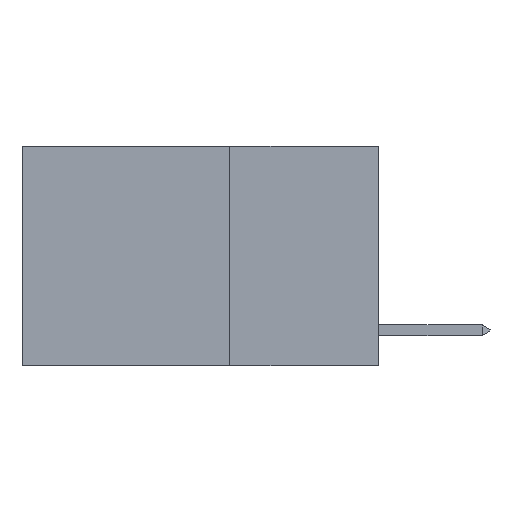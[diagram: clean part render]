
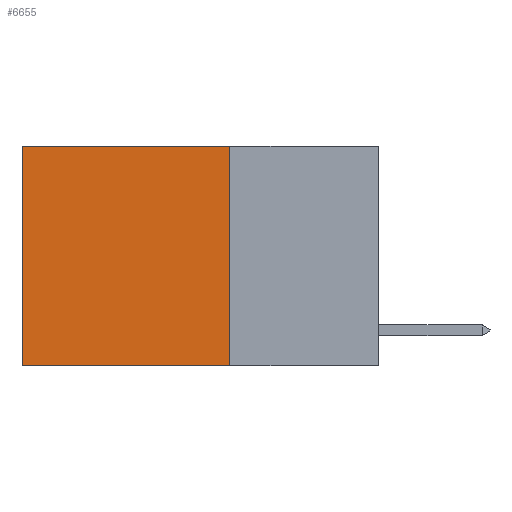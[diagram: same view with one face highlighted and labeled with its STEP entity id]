
A CAD part, left-side view. The second image highlights one B-rep face of the part: STEP entity #6655.
In plain terms, the highlighted planar face has unit normal (-1, 0, 0).
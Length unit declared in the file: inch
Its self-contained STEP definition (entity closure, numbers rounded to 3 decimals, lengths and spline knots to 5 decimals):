
#853 = EDGE_CURVE ( 'NONE', #12698, #9945, #14591, .T. ) ;
#1977 = CARTESIAN_POINT ( 'NONE',  ( 0.2625, 0.25, 0. ) ) ;
#3309 = VECTOR ( 'NONE', #4753, 39.37008 ) ;
#3991 = ORIENTED_EDGE ( 'NONE', *, *, #853, .F. ) ;
#4753 = DIRECTION ( 'NONE',  ( 0., 0., -1. ) ) ;
#4944 = CARTESIAN_POINT ( 'NONE',  ( 0.2625, 0.25, 0. ) ) ;
#5026 = VECTOR ( 'NONE', #20307, 39.37008 ) ;
#5047 = VERTEX_POINT ( 'NONE', #17687 ) ;
#5122 = VECTOR ( 'NONE', #18164, 39.37008 ) ;
#6655 = ADVANCED_FACE ( 'NONE', ( #19489 ), #18975, .F. ) ;
#7430 = VERTEX_POINT ( 'NONE', #4944 ) ;
#7763 = AXIS2_PLACEMENT_3D ( 'NONE', #10168, #20741, #10244 ) ;
#9034 = CARTESIAN_POINT ( 'NONE',  ( 0.2625, 0.6, -0.37 ) ) ;
#9945 = VERTEX_POINT ( 'NONE', #9034 ) ;
#10168 = CARTESIAN_POINT ( 'NONE',  ( 0.2625, 0.25, 0. ) ) ;
#10244 = DIRECTION ( 'NONE',  ( 0., 0., -1. ) ) ;
#10318 = CARTESIAN_POINT ( 'NONE',  ( 0.2625, 0.25, -0.37 ) ) ;
#11488 = EDGE_CURVE ( 'NONE', #7430, #12698, #12929, .T. ) ;
#12698 = VERTEX_POINT ( 'NONE', #10318 ) ;
#12855 = LINE ( 'NONE', #1977, #22154 ) ;
#12929 = LINE ( 'NONE', #17194, #3309 ) ;
#14591 = LINE ( 'NONE', #18290, #5122 ) ;
#14616 = DIRECTION ( 'NONE',  ( 0., 1., 0. ) ) ;
#15682 = ORIENTED_EDGE ( 'NONE', *, *, #22664, .T. ) ;
#17194 = CARTESIAN_POINT ( 'NONE',  ( 0.2625, 0.25, 0. ) ) ;
#17683 = EDGE_LOOP ( 'NONE', ( #22418, #3991, #19879, #15682 ) ) ;
#17687 = CARTESIAN_POINT ( 'NONE',  ( 0.2625, 0.6, 0. ) ) ;
#18164 = DIRECTION ( 'NONE',  ( 0., 1., 0. ) ) ;
#18290 = CARTESIAN_POINT ( 'NONE',  ( 0.2625, 0.25, -0.37 ) ) ;
#18566 = CARTESIAN_POINT ( 'NONE',  ( 0.2625, 0.6, 0. ) ) ;
#18975 = PLANE ( 'NONE',  #7763 ) ;
#19161 = LINE ( 'NONE', #18566, #5026 ) ;
#19489 = FACE_OUTER_BOUND ( 'NONE', #17683, .T. ) ;
#19879 = ORIENTED_EDGE ( 'NONE', *, *, #11488, .F. ) ;
#20307 = DIRECTION ( 'NONE',  ( 0., 0., -1. ) ) ;
#20741 = DIRECTION ( 'NONE',  ( 1., 0., 0. ) ) ;
#22100 = EDGE_CURVE ( 'NONE', #5047, #9945, #19161, .T. ) ;
#22154 = VECTOR ( 'NONE', #14616, 39.37008 ) ;
#22418 = ORIENTED_EDGE ( 'NONE', *, *, #22100, .T. ) ;
#22664 = EDGE_CURVE ( 'NONE', #7430, #5047, #12855, .T. ) ;
